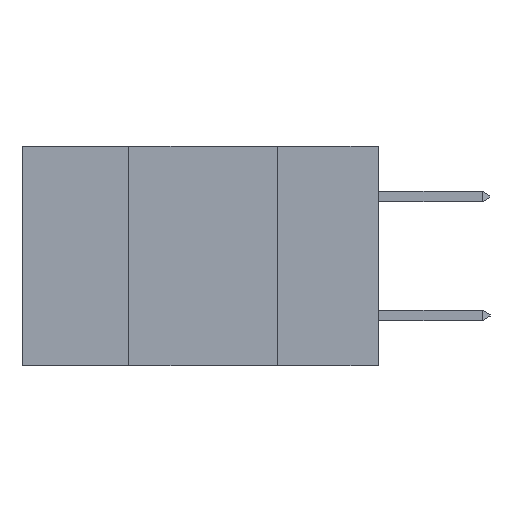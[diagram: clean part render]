
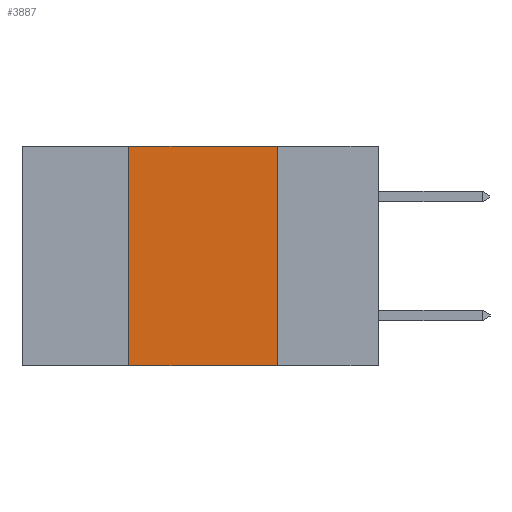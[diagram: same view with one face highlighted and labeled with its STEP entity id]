
A CAD part, left-side view. The second image highlights one B-rep face of the part: STEP entity #3887.
In plain terms, the highlighted planar face has unit normal (-1, 0, 0).
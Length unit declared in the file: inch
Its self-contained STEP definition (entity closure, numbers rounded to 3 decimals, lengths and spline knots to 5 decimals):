
#259 = PLANE ( 'NONE',  #6515 ) ;
#517 = EDGE_LOOP ( 'NONE', ( #1980, #10877, #6611, #3151 ) ) ;
#977 = LINE ( 'NONE', #2451, #11560 ) ;
#978 = EDGE_CURVE ( 'NONE', #7377, #8831, #13272, .T. ) ;
#1099 = CARTESIAN_POINT ( 'NONE',  ( 0., 0.42, -0.37 ) ) ;
#1187 = DIRECTION ( 'NONE',  ( 0., 0., -1. ) ) ;
#1340 = DIRECTION ( 'NONE',  ( 1., 0., 0. ) ) ;
#1369 = CARTESIAN_POINT ( 'NONE',  ( 0., 0.6, 0. ) ) ;
#1980 = ORIENTED_EDGE ( 'NONE', *, *, #13679, .F. ) ;
#2451 = CARTESIAN_POINT ( 'NONE',  ( 0., 0.6, -0.37 ) ) ;
#2563 = LINE ( 'NONE', #10421, #11034 ) ;
#2712 = DIRECTION ( 'NONE',  ( 0., -1., 0. ) ) ;
#3006 = VERTEX_POINT ( 'NONE', #8074 ) ;
#3151 = ORIENTED_EDGE ( 'NONE', *, *, #7869, .T. ) ;
#3760 = FACE_OUTER_BOUND ( 'NONE', #517, .T. ) ;
#3841 = EDGE_CURVE ( 'NONE', #8831, #10028, #4114, .T. ) ;
#3887 = ADVANCED_FACE ( 'NONE', ( #3760 ), #259, .F. ) ;
#4114 = LINE ( 'NONE', #11065, #9708 ) ;
#4714 = VECTOR ( 'NONE', #8553, 39.37008 ) ;
#6515 = AXIS2_PLACEMENT_3D ( 'NONE', #1369, #1340, #1187 ) ;
#6611 = ORIENTED_EDGE ( 'NONE', *, *, #978, .F. ) ;
#7068 = CARTESIAN_POINT ( 'NONE',  ( 0., 0.42, -0.37 ) ) ;
#7377 = VERTEX_POINT ( 'NONE', #1099 ) ;
#7752 = CARTESIAN_POINT ( 'NONE',  ( 0., 0.42, 0. ) ) ;
#7869 = EDGE_CURVE ( 'NONE', #7377, #3006, #977, .T. ) ;
#8074 = CARTESIAN_POINT ( 'NONE',  ( 0., 0.17, -0.37 ) ) ;
#8553 = DIRECTION ( 'NONE',  ( 0., 0., 1. ) ) ;
#8831 = VERTEX_POINT ( 'NONE', #7752 ) ;
#9236 = CARTESIAN_POINT ( 'NONE',  ( 0., 0.17, 0. ) ) ;
#9708 = VECTOR ( 'NONE', #10896, 39.37008 ) ;
#10028 = VERTEX_POINT ( 'NONE', #9236 ) ;
#10401 = DIRECTION ( 'NONE',  ( 0., 0., -1. ) ) ;
#10421 = CARTESIAN_POINT ( 'NONE',  ( 0., 0.17, -0.37 ) ) ;
#10877 = ORIENTED_EDGE ( 'NONE', *, *, #3841, .F. ) ;
#10896 = DIRECTION ( 'NONE',  ( 0., -1., 0. ) ) ;
#11034 = VECTOR ( 'NONE', #10401, 39.37008 ) ;
#11065 = CARTESIAN_POINT ( 'NONE',  ( 0., 0.6, 0. ) ) ;
#11560 = VECTOR ( 'NONE', #2712, 39.37008 ) ;
#13272 = LINE ( 'NONE', #7068, #4714 ) ;
#13679 = EDGE_CURVE ( 'NONE', #10028, #3006, #2563, .T. ) ;
